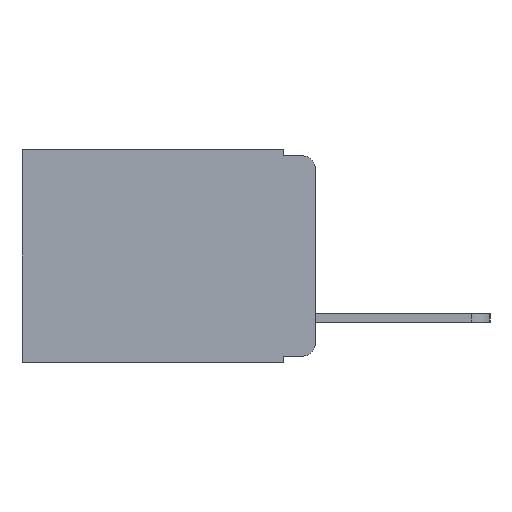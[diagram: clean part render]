
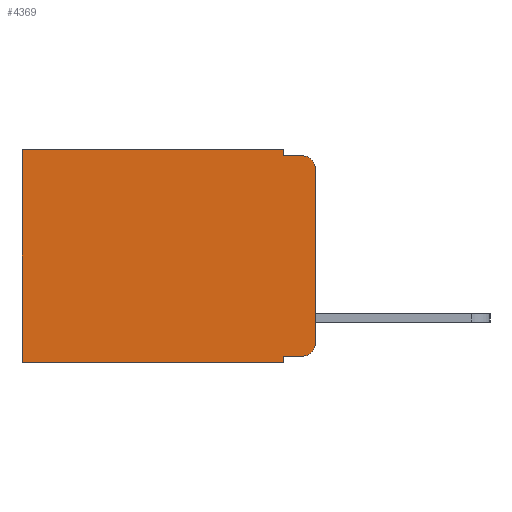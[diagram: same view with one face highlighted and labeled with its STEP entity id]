
A CAD part, left-side view. The second image highlights one B-rep face of the part: STEP entity #4369.
In plain terms, the highlighted planar face has unit normal (-1, 0, 0).
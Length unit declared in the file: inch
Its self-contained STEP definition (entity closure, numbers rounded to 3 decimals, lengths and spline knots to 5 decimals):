
#167 = VERTEX_POINT ( 'NONE', #12984 ) ;
#745 = DIRECTION ( 'NONE',  ( 0., -1., 0. ) ) ;
#1057 = CIRCLE ( 'NONE', #6032, 0.02 ) ;
#1432 = DIRECTION ( 'NONE',  ( 0., 1., 0. ) ) ;
#1503 = CARTESIAN_POINT ( 'NONE',  ( 0.298, 0., -0.313 ) ) ;
#2028 = VECTOR ( 'NONE', #745, 39.37008 ) ;
#2330 = VERTEX_POINT ( 'NONE', #7465 ) ;
#2575 = CARTESIAN_POINT ( 'NONE',  ( 0.298, 0.051, -0.01 ) ) ;
#2621 = DIRECTION ( 'NONE',  ( -1., 0., 0. ) ) ;
#2896 = EDGE_CURVE ( 'NONE', #6966, #7038, #3784, .T. ) ;
#2901 = VERTEX_POINT ( 'NONE', #8667 ) ;
#2961 = DIRECTION ( 'NONE',  ( 0., 0., -1. ) ) ;
#3199 = VERTEX_POINT ( 'NONE', #1503 ) ;
#3489 = DIRECTION ( 'NONE',  ( 0., -1., 0. ) ) ;
#3727 = LINE ( 'NONE', #12991, #11055 ) ;
#3743 = CARTESIAN_POINT ( 'NONE',  ( 0.298, 0.473, 0. ) ) ;
#3749 = VERTEX_POINT ( 'NONE', #6892 ) ;
#3784 = LINE ( 'NONE', #5138, #12740 ) ;
#4022 = CARTESIAN_POINT ( 'NONE',  ( 0.298, 0., -0.03 ) ) ;
#4076 = DIRECTION ( 'NONE',  ( 0., 0., -1. ) ) ;
#4369 = ADVANCED_FACE ( 'NONE', ( #11545 ), #6250, .F. ) ;
#4595 = EDGE_CURVE ( 'NONE', #12167, #3199, #3727, .T. ) ;
#4824 = CARTESIAN_POINT ( 'NONE',  ( 0.298, 0., 0. ) ) ;
#4944 = CARTESIAN_POINT ( 'NONE',  ( 0.298, 0., -0.343 ) ) ;
#5138 = CARTESIAN_POINT ( 'NONE',  ( 0.298, 0., 0. ) ) ;
#5503 = LINE ( 'NONE', #13529, #2028 ) ;
#6032 = AXIS2_PLACEMENT_3D ( 'NONE', #7374, #7404, #11989 ) ;
#6132 = EDGE_CURVE ( 'NONE', #10441, #167, #5503, .T. ) ;
#6250 = PLANE ( 'NONE',  #14081 ) ;
#6710 = CARTESIAN_POINT ( 'NONE',  ( 0.298, 0.02, -0.333 ) ) ;
#6814 = VERTEX_POINT ( 'NONE', #6710 ) ;
#6881 = EDGE_CURVE ( 'NONE', #12167, #167, #1057, .T. ) ;
#6892 = CARTESIAN_POINT ( 'NONE',  ( 0.298, 0.051, -0.343 ) ) ;
#6920 = CARTESIAN_POINT ( 'NONE',  ( 0.298, 0.051, -0.333 ) ) ;
#6966 = VERTEX_POINT ( 'NONE', #8787 ) ;
#7038 = VERTEX_POINT ( 'NONE', #10381 ) ;
#7374 = CARTESIAN_POINT ( 'NONE',  ( 0.298, 0.02, -0.03 ) ) ;
#7404 = DIRECTION ( 'NONE',  ( -1., 0., 0. ) ) ;
#7465 = CARTESIAN_POINT ( 'NONE',  ( 0.298, 0.051, -0.333 ) ) ;
#7513 = VECTOR ( 'NONE', #10064, 39.37008 ) ;
#7518 = LINE ( 'NONE', #3743, #13095 ) ;
#7682 = EDGE_CURVE ( 'NONE', #3749, #2901, #10339, .T. ) ;
#8119 = DIRECTION ( 'NONE',  ( 0., 0., -1. ) ) ;
#8212 = LINE ( 'NONE', #10336, #13433 ) ;
#8340 = EDGE_CURVE ( 'NONE', #7038, #2901, #7518, .T. ) ;
#8667 = CARTESIAN_POINT ( 'NONE',  ( 0.298, 0.473, -0.343 ) ) ;
#8787 = CARTESIAN_POINT ( 'NONE',  ( 0.298, 0.051, 0. ) ) ;
#9335 = CARTESIAN_POINT ( 'NONE',  ( 0.298, 0.02, -0.313 ) ) ;
#9680 = VECTOR ( 'NONE', #3489, 39.37008 ) ;
#9745 = EDGE_CURVE ( 'NONE', #6966, #10441, #13013, .T. ) ;
#9945 = VECTOR ( 'NONE', #8119, 39.37008 ) ;
#10064 = DIRECTION ( 'NONE',  ( 0., 1., 0. ) ) ;
#10225 = CARTESIAN_POINT ( 'NONE',  ( 0.298, 0.051, 0. ) ) ;
#10336 = CARTESIAN_POINT ( 'NONE',  ( 0.298, 0.051, 0. ) ) ;
#10339 = LINE ( 'NONE', #4944, #7513 ) ;
#10369 = DIRECTION ( 'NONE',  ( 0., 0., -1. ) ) ;
#10381 = CARTESIAN_POINT ( 'NONE',  ( 0.298, 0.473, 0. ) ) ;
#10441 = VERTEX_POINT ( 'NONE', #2575 ) ;
#10912 = DIRECTION ( 'NONE',  ( 0., 0., -1. ) ) ;
#11055 = VECTOR ( 'NONE', #2961, 39.37008 ) ;
#11151 = DIRECTION ( 'NONE',  ( 1., 0., 0. ) ) ;
#11363 = DIRECTION ( 'NONE',  ( 0., 0., -1. ) ) ;
#11545 = FACE_OUTER_BOUND ( 'NONE', #14004, .T. ) ;
#11563 = EDGE_CURVE ( 'NONE', #6814, #3199, #11657, .T. ) ;
#11657 = CIRCLE ( 'NONE', #12656, 0.02 ) ;
#11989 = DIRECTION ( 'NONE',  ( 0., 0., -1. ) ) ;
#12167 = VERTEX_POINT ( 'NONE', #4022 ) ;
#12210 = ORIENTED_EDGE ( 'NONE', *, *, #4595, .F. ) ;
#12242 = ORIENTED_EDGE ( 'NONE', *, *, #6132, .F. ) ;
#12297 = ORIENTED_EDGE ( 'NONE', *, *, #6881, .T. ) ;
#12355 = ORIENTED_EDGE ( 'NONE', *, *, #2896, .T. ) ;
#12454 = ORIENTED_EDGE ( 'NONE', *, *, #9745, .F. ) ;
#12545 = ORIENTED_EDGE ( 'NONE', *, *, #7682, .F. ) ;
#12592 = ORIENTED_EDGE ( 'NONE', *, *, #8340, .T. ) ;
#12608 = ORIENTED_EDGE ( 'NONE', *, *, #13780, .T. ) ;
#12656 = AXIS2_PLACEMENT_3D ( 'NONE', #9335, #2621, #10369 ) ;
#12716 = ORIENTED_EDGE ( 'NONE', *, *, #13248, .F. ) ;
#12740 = VECTOR ( 'NONE', #1432, 39.37008 ) ;
#12750 = LINE ( 'NONE', #6920, #9680 ) ;
#12808 = ORIENTED_EDGE ( 'NONE', *, *, #11563, .T. ) ;
#12984 = CARTESIAN_POINT ( 'NONE',  ( 0.298, 0.02, -0.01 ) ) ;
#12991 = CARTESIAN_POINT ( 'NONE',  ( 0.298, 0., 0. ) ) ;
#13013 = LINE ( 'NONE', #10225, #9945 ) ;
#13095 = VECTOR ( 'NONE', #4076, 39.37008 ) ;
#13248 = EDGE_CURVE ( 'NONE', #2330, #3749, #8212, .T. ) ;
#13433 = VECTOR ( 'NONE', #11363, 39.37008 ) ;
#13529 = CARTESIAN_POINT ( 'NONE',  ( 0.298, 0.051, -0.01 ) ) ;
#13780 = EDGE_CURVE ( 'NONE', #2330, #6814, #12750, .T. ) ;
#14004 = EDGE_LOOP ( 'NONE', ( #12210, #12297, #12242, #12454, #12355, #12592, #12545, #12716, #12608, #12808 ) ) ;
#14081 = AXIS2_PLACEMENT_3D ( 'NONE', #4824, #11151, #10912 ) ;
